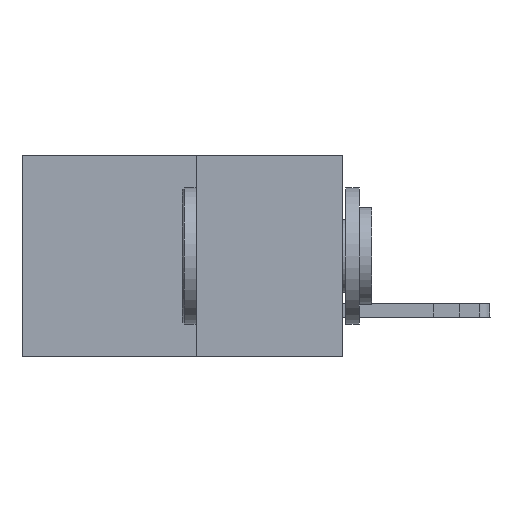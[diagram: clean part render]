
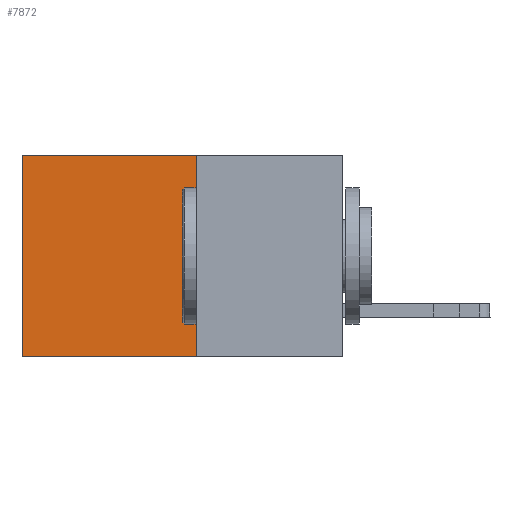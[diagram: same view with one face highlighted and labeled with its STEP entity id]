
A CAD part, left-side view. The second image highlights one B-rep face of the part: STEP entity #7872.
In plain terms, the highlighted planar face has unit normal (-1, 0, 0).
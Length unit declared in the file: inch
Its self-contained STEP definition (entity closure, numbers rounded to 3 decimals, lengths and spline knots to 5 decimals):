
#73 = CARTESIAN_POINT ( 'NONE',  ( 0.277, 0.59, 0. ) ) ;
#1998 = AXIS2_PLACEMENT_3D ( 'NONE', #3052, #13749, #11471 ) ;
#2381 = CARTESIAN_POINT ( 'NONE',  ( 0.277, 0.27, -0.37 ) ) ;
#2786 = CARTESIAN_POINT ( 'NONE',  ( 0.277, 0.59, -0.37 ) ) ;
#2803 = VERTEX_POINT ( 'NONE', #14935 ) ;
#3052 = CARTESIAN_POINT ( 'NONE',  ( 0.277, 0.27, -0.37 ) ) ;
#3084 = EDGE_CURVE ( 'NONE', #3879, #4458, #4040, .T. ) ;
#3879 = VERTEX_POINT ( 'NONE', #73 ) ;
#3998 = ORIENTED_EDGE ( 'NONE', *, *, #3084, .T. ) ;
#4011 = CARTESIAN_POINT ( 'NONE',  ( 0.277, 0.27, -0.37 ) ) ;
#4040 = LINE ( 'NONE', #2786, #10637 ) ;
#4458 = VERTEX_POINT ( 'NONE', #5542 ) ;
#4983 = DIRECTION ( 'NONE',  ( 0., 0., -1. ) ) ;
#5542 = CARTESIAN_POINT ( 'NONE',  ( 0.277, 0.59, -0.37 ) ) ;
#6608 = ORIENTED_EDGE ( 'NONE', *, *, #10939, .F. ) ;
#6981 = EDGE_CURVE ( 'NONE', #9053, #3879, #14163, .T. ) ;
#7872 = ADVANCED_FACE ( 'NONE', ( #14053 ), #15006, .F. ) ;
#8204 = VECTOR ( 'NONE', #11676, 39.37008 ) ;
#8737 = DIRECTION ( 'NONE',  ( 0., 0., -1. ) ) ;
#9053 = VERTEX_POINT ( 'NONE', #10166 ) ;
#9064 = DIRECTION ( 'NONE',  ( 0., 1., 0. ) ) ;
#9479 = ORIENTED_EDGE ( 'NONE', *, *, #14292, .F. ) ;
#10166 = CARTESIAN_POINT ( 'NONE',  ( 0.277, 0.27, 0. ) ) ;
#10620 = VECTOR ( 'NONE', #8737, 39.37008 ) ;
#10637 = VECTOR ( 'NONE', #4983, 39.37008 ) ;
#10939 = EDGE_CURVE ( 'NONE', #2803, #4458, #13157, .T. ) ;
#11178 = LINE ( 'NONE', #4011, #10620 ) ;
#11471 = DIRECTION ( 'NONE',  ( 0., 0., -1. ) ) ;
#11676 = DIRECTION ( 'NONE',  ( 0., 1., 0. ) ) ;
#13036 = EDGE_LOOP ( 'NONE', ( #3998, #6608, #9479, #13571 ) ) ;
#13157 = LINE ( 'NONE', #2381, #8204 ) ;
#13571 = ORIENTED_EDGE ( 'NONE', *, *, #6981, .T. ) ;
#13749 = DIRECTION ( 'NONE',  ( 1., 0., 0. ) ) ;
#14053 = FACE_OUTER_BOUND ( 'NONE', #13036, .T. ) ;
#14083 = CARTESIAN_POINT ( 'NONE',  ( 0.277, 0.27, 0. ) ) ;
#14163 = LINE ( 'NONE', #14083, #14987 ) ;
#14292 = EDGE_CURVE ( 'NONE', #9053, #2803, #11178, .T. ) ;
#14935 = CARTESIAN_POINT ( 'NONE',  ( 0.277, 0.27, -0.37 ) ) ;
#14987 = VECTOR ( 'NONE', #9064, 39.37008 ) ;
#15006 = PLANE ( 'NONE',  #1998 ) ;
